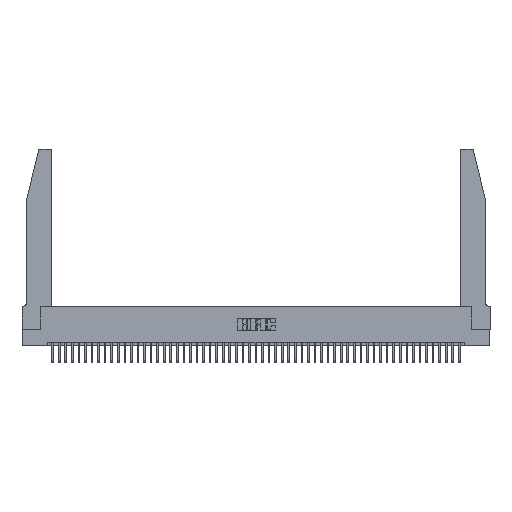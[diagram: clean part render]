
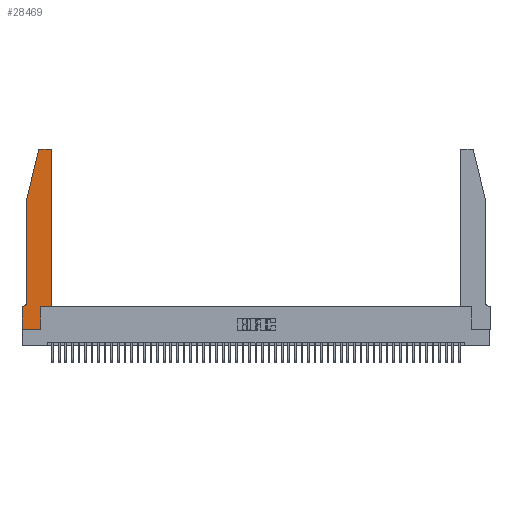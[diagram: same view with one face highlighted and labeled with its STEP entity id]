
A CAD part, top view. The second image highlights one B-rep face of the part: STEP entity #28469.
In plain terms, the highlighted planar face has unit normal (0, 0, 1).
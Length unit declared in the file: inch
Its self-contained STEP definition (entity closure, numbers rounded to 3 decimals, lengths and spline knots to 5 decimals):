
#334 = DIRECTION ( 'NONE',  ( 0., 0., 1. ) ) ;
#338 = AXIS2_PLACEMENT_3D ( 'NONE', #10332, #23051, #43636 ) ;
#1066 = EDGE_CURVE ( 'NONE', #14734, #36284, #19563, .T. ) ;
#1933 = LINE ( 'NONE', #50661, #14792 ) ;
#2709 = ORIENTED_EDGE ( 'NONE', *, *, #19165, .T. ) ;
#2737 = DIRECTION ( 'NONE',  ( 1., 0., 0. ) ) ;
#3867 = CIRCLE ( 'NONE', #42785, 0.03 ) ;
#6221 = ORIENTED_EDGE ( 'NONE', *, *, #19586, .T. ) ;
#6520 = DIRECTION ( 'NONE',  ( 0., 1., 0. ) ) ;
#6683 = AXIS2_PLACEMENT_3D ( 'NONE', #29055, #8769, #25631 ) ;
#6742 = CARTESIAN_POINT ( 'NONE',  ( 0., 0.35, 0.37 ) ) ;
#7081 = CIRCLE ( 'NONE', #23895, 0.03 ) ;
#7226 = DIRECTION ( 'NONE',  ( 0., 1., 0. ) ) ;
#7669 = LINE ( 'NONE', #44147, #17355 ) ;
#8746 = DIRECTION ( 'NONE',  ( 0., -1., 0. ) ) ;
#8769 = DIRECTION ( 'NONE',  ( 0., 0., -1. ) ) ;
#8852 = LINE ( 'NONE', #33171, #46016 ) ;
#9796 = VERTEX_POINT ( 'NONE', #51556 ) ;
#10101 = CARTESIAN_POINT ( 'NONE',  ( 0.2865, 0., 0.37 ) ) ;
#10332 = CARTESIAN_POINT ( 'NONE',  ( 0., 0.35, 0.37 ) ) ;
#11070 = LINE ( 'NONE', #45618, #23251 ) ;
#11439 = CARTESIAN_POINT ( 'NONE',  ( 0.0755, 2., 0.37 ) ) ;
#11496 = DIRECTION ( 'NONE',  ( 1., 0., 0. ) ) ;
#12354 = EDGE_CURVE ( 'NONE', #28176, #37202, #11070, .T. ) ;
#14200 = ORIENTED_EDGE ( 'NONE', *, *, #24059, .T. ) ;
#14734 = VERTEX_POINT ( 'NONE', #29920 ) ;
#14792 = VECTOR ( 'NONE', #46584, 39.37008 ) ;
#15049 = CIRCLE ( 'NONE', #6683, 0.07 ) ;
#15080 = VECTOR ( 'NONE', #11496, 39.37008 ) ;
#15124 = CARTESIAN_POINT ( 'NONE',  ( 0.4205, 2.72, 0.37 ) ) ;
#15319 = CARTESIAN_POINT ( 'NONE',  ( 0.4505, 0.35, 0.37 ) ) ;
#16083 = LINE ( 'NONE', #16144, #32747 ) ;
#16144 = CARTESIAN_POINT ( 'NONE',  ( 0.0755, 0.35, 0.37 ) ) ;
#16619 = VECTOR ( 'NONE', #8746, 39.37008 ) ;
#16827 = CARTESIAN_POINT ( 'NONE',  ( 0.284, 2.75, 0.37 ) ) ;
#17355 = VECTOR ( 'NONE', #6520, 39.37008 ) ;
#18420 = DIRECTION ( 'NONE',  ( 0., -1., 0. ) ) ;
#18695 = DIRECTION ( 'NONE',  ( 0., 0., 1. ) ) ;
#19084 = EDGE_LOOP ( 'NONE', ( #44290, #48038, #47120, #40774, #22369, #2709, #39633, #29005, #37873, #35436, #6221, #14200 ) ) ;
#19165 = EDGE_CURVE ( 'NONE', #9796, #48160, #16083, .T. ) ;
#19172 = EDGE_CURVE ( 'NONE', #42563, #52647, #3867, .T. ) ;
#19563 = LINE ( 'NONE', #22020, #15080 ) ;
#19586 = EDGE_CURVE ( 'NONE', #37202, #35806, #26361, .T. ) ;
#19649 = EDGE_CURVE ( 'NONE', #36284, #28176, #7669, .T. ) ;
#20052 = EDGE_CURVE ( 'NONE', #46838, #42563, #1933, .T. ) ;
#22020 = CARTESIAN_POINT ( 'NONE',  ( 0., 0., 0.37 ) ) ;
#22369 = ORIENTED_EDGE ( 'NONE', *, *, #33645, .T. ) ;
#23051 = DIRECTION ( 'NONE',  ( 0., 0., 1. ) ) ;
#23251 = VECTOR ( 'NONE', #50585, 39.37008 ) ;
#23895 = AXIS2_PLACEMENT_3D ( 'NONE', #15124, #18695, #2737 ) ;
#24008 = FACE_OUTER_BOUND ( 'NONE', #19084, .T. ) ;
#24059 = EDGE_CURVE ( 'NONE', #35806, #46838, #7081, .T. ) ;
#25049 = CARTESIAN_POINT ( 'NONE',  ( 0.2865, 0.35, 0.37 ) ) ;
#25631 = DIRECTION ( 'NONE',  ( -1., 0., 0. ) ) ;
#26361 = LINE ( 'NONE', #15319, #41719 ) ;
#27186 = CARTESIAN_POINT ( 'NONE',  ( 0.4505, 2.72, 0.37 ) ) ;
#28176 = VERTEX_POINT ( 'NONE', #25049 ) ;
#28469 = ADVANCED_FACE ( 'NONE', ( #24008 ), #47550, .T. ) ;
#29005 = ORIENTED_EDGE ( 'NONE', *, *, #1066, .T. ) ;
#29027 = CARTESIAN_POINT ( 'NONE',  ( 0.284, 2.72, 0.37 ) ) ;
#29055 = CARTESIAN_POINT ( 'NONE',  ( 0.0055, 0.42, 0.37 ) ) ;
#29920 = CARTESIAN_POINT ( 'NONE',  ( 0., 0., 0.37 ) ) ;
#32747 = VECTOR ( 'NONE', #40823, 39.37008 ) ;
#33171 = CARTESIAN_POINT ( 'NONE',  ( 0.0755, 2., 0.37 ) ) ;
#33348 = DIRECTION ( 'NONE',  ( 1., 0., 0. ) ) ;
#33645 = EDGE_CURVE ( 'NONE', #36317, #9796, #15049, .T. ) ;
#35311 = CARTESIAN_POINT ( 'NONE',  ( 0., 0., 0.37 ) ) ;
#35436 = ORIENTED_EDGE ( 'NONE', *, *, #12354, .T. ) ;
#35806 = VERTEX_POINT ( 'NONE', #27186 ) ;
#35818 = VERTEX_POINT ( 'NONE', #11439 ) ;
#36284 = VERTEX_POINT ( 'NONE', #10101 ) ;
#36317 = VERTEX_POINT ( 'NONE', #41989 ) ;
#37202 = VERTEX_POINT ( 'NONE', #43043 ) ;
#37873 = ORIENTED_EDGE ( 'NONE', *, *, #19649, .T. ) ;
#37967 = CARTESIAN_POINT ( 'NONE',  ( 0.0755, 2., 0.37 ) ) ;
#39633 = ORIENTED_EDGE ( 'NONE', *, *, #48231, .T. ) ;
#40246 = EDGE_CURVE ( 'NONE', #52647, #35818, #8852, .T. ) ;
#40774 = ORIENTED_EDGE ( 'NONE', *, *, #42724, .T. ) ;
#40823 = DIRECTION ( 'NONE',  ( -1., 0., 0. ) ) ;
#41719 = VECTOR ( 'NONE', #7226, 39.37008 ) ;
#41989 = CARTESIAN_POINT ( 'NONE',  ( 0.0755, 0.42, 0.37 ) ) ;
#42112 = CARTESIAN_POINT ( 'NONE',  ( 0.25487, 2.72718, 0.37 ) ) ;
#42563 = VERTEX_POINT ( 'NONE', #16827 ) ;
#42724 = EDGE_CURVE ( 'NONE', #35818, #36317, #43552, .T. ) ;
#42785 = AXIS2_PLACEMENT_3D ( 'NONE', #29027, #334, #33348 ) ;
#43043 = CARTESIAN_POINT ( 'NONE',  ( 0.4505, 0.35, 0.37 ) ) ;
#43552 = LINE ( 'NONE', #37967, #16619 ) ;
#43636 = DIRECTION ( 'NONE',  ( 1., 0., 0. ) ) ;
#44147 = CARTESIAN_POINT ( 'NONE',  ( 0.2865, 0.35, 0.37 ) ) ;
#44290 = ORIENTED_EDGE ( 'NONE', *, *, #20052, .T. ) ;
#45618 = CARTESIAN_POINT ( 'NONE',  ( 0.4505, 0.35, 0.37 ) ) ;
#45626 = DIRECTION ( 'NONE',  ( -0.239, -0.971, 0. ) ) ;
#46016 = VECTOR ( 'NONE', #45626, 39.37008 ) ;
#46344 = LINE ( 'NONE', #35311, #48271 ) ;
#46377 = CARTESIAN_POINT ( 'NONE',  ( 0.4205, 2.75, 0.37 ) ) ;
#46584 = DIRECTION ( 'NONE',  ( -1., 0., 0. ) ) ;
#46838 = VERTEX_POINT ( 'NONE', #46377 ) ;
#47120 = ORIENTED_EDGE ( 'NONE', *, *, #40246, .T. ) ;
#47550 = PLANE ( 'NONE',  #338 ) ;
#48038 = ORIENTED_EDGE ( 'NONE', *, *, #19172, .T. ) ;
#48160 = VERTEX_POINT ( 'NONE', #6742 ) ;
#48231 = EDGE_CURVE ( 'NONE', #48160, #14734, #46344, .T. ) ;
#48271 = VECTOR ( 'NONE', #18420, 39.37008 ) ;
#50585 = DIRECTION ( 'NONE',  ( 1., 0., 0. ) ) ;
#50661 = CARTESIAN_POINT ( 'NONE',  ( 0.2605, 2.75, 0.37 ) ) ;
#51556 = CARTESIAN_POINT ( 'NONE',  ( 0.0055, 0.35, 0.37 ) ) ;
#52647 = VERTEX_POINT ( 'NONE', #42112 ) ;
